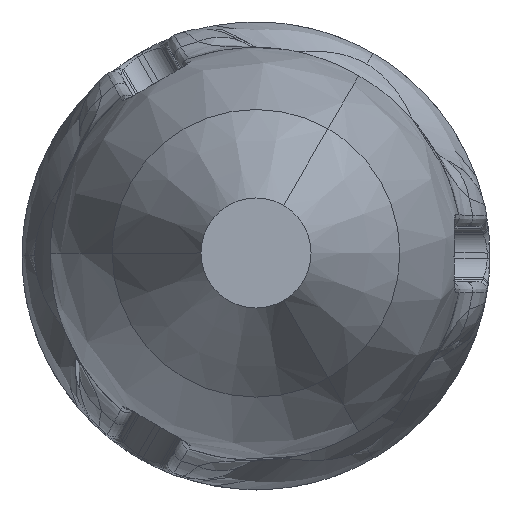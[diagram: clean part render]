
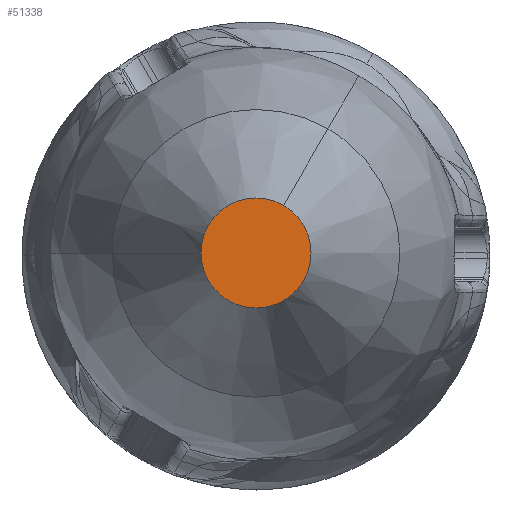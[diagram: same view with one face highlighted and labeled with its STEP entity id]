
A CAD part, top view. The second image highlights one B-rep face of the part: STEP entity #51338.
In plain terms, the highlighted planar face has unit normal (0, 0, 1).
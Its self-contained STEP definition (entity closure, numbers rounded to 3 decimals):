
#40723 = CONICAL_SURFACE('',#40724,15.,0.43);
#40724 = AXIS2_PLACEMENT_3D('',#40725,#40726,#40727);
#40725 = CARTESIAN_POINT('',(0.,0.,105.));
#40726 = DIRECTION('',(0.,0.,-1.));
#40727 = DIRECTION('',(-0.5,0.866,0.));
#42146 = CONICAL_SURFACE('',#42147,15.,0.43);
#42147 = AXIS2_PLACEMENT_3D('',#42148,#42149,#42150);
#42148 = CARTESIAN_POINT('',(0.,0.,105.));
#42149 = DIRECTION('',(0.,0.,-1.));
#42150 = DIRECTION('',(-0.5,-0.866,0.));
#47327 = CONICAL_SURFACE('',#47328,15.,0.43);
#47328 = AXIS2_PLACEMENT_3D('',#47329,#47330,#47331);
#47329 = CARTESIAN_POINT('',(0.,0.,105.));
#47330 = DIRECTION('',(-0.,0.,-1.));
#47331 = DIRECTION('',(1.,0.,0.));
#47983 = VERTEX_POINT('',#47984);
#47984 = CARTESIAN_POINT('',(-4.,0.,129.));
#48005 = VERTEX_POINT('',#48006);
#48006 = CARTESIAN_POINT('',(2.,-3.464,129.));
#48025 = EDGE_CURVE('',#47983,#48005,#48026,.T.);
#48026 = SURFACE_CURVE('',#48027,(#48032,#48039),.PCURVE_S1.);
#48027 = CIRCLE('',#48028,4.);
#48028 = AXIS2_PLACEMENT_3D('',#48029,#48030,#48031);
#48029 = CARTESIAN_POINT('',(0.,0.,129.));
#48030 = DIRECTION('',(0.,0.,1.));
#48031 = DIRECTION('',(-0.5,0.866,0.));
#48032 = PCURVE('',#40723,#48033);
#48033 = DEFINITIONAL_REPRESENTATION('',(#48034),#48038);
#48034 = LINE('',#48035,#48036);
#48035 = CARTESIAN_POINT('',(-0.,-24.));
#48036 = VECTOR('',#48037,1.);
#48037 = DIRECTION('',(-1.,-0.));
#48038 = ( GEOMETRIC_REPRESENTATION_CONTEXT(2) 
PARAMETRIC_REPRESENTATION_CONTEXT() REPRESENTATION_CONTEXT('2D SPACE',''
  ) );
#48039 = PCURVE('',#48040,#48045);
#48040 = PLANE('',#48041);
#48041 = AXIS2_PLACEMENT_3D('',#48042,#48043,#48044);
#48042 = CARTESIAN_POINT('',(0.,0.,129.));
#48043 = DIRECTION('',(0.,0.,1.));
#48044 = DIRECTION('',(0.,1.,0.));
#48045 = DEFINITIONAL_REPRESENTATION('',(#48046),#48050);
#48046 = CIRCLE('',#48047,4.);
#48047 = AXIS2_PLACEMENT_2D('',#48048,#48049);
#48048 = CARTESIAN_POINT('',(0.,0.));
#48049 = DIRECTION('',(0.866,0.5));
#48050 = ( GEOMETRIC_REPRESENTATION_CONTEXT(2) 
PARAMETRIC_REPRESENTATION_CONTEXT() REPRESENTATION_CONTEXT('2D SPACE',''
  ) );
#48536 = VERTEX_POINT('',#48537);
#48537 = CARTESIAN_POINT('',(2.,3.464,129.));
#48556 = EDGE_CURVE('',#48005,#48536,#48557,.T.);
#48557 = SURFACE_CURVE('',#48558,(#48563,#48570),.PCURVE_S1.);
#48558 = CIRCLE('',#48559,4.);
#48559 = AXIS2_PLACEMENT_3D('',#48560,#48561,#48562);
#48560 = CARTESIAN_POINT('',(0.,0.,129.));
#48561 = DIRECTION('',(0.,0.,1.));
#48562 = DIRECTION('',(-0.5,-0.866,0.));
#48563 = PCURVE('',#42146,#48564);
#48564 = DEFINITIONAL_REPRESENTATION('',(#48565),#48569);
#48565 = LINE('',#48566,#48567);
#48566 = CARTESIAN_POINT('',(-0.,-24.));
#48567 = VECTOR('',#48568,1.);
#48568 = DIRECTION('',(-1.,-0.));
#48569 = ( GEOMETRIC_REPRESENTATION_CONTEXT(2) 
PARAMETRIC_REPRESENTATION_CONTEXT() REPRESENTATION_CONTEXT('2D SPACE',''
  ) );
#48570 = PCURVE('',#48040,#48571);
#48571 = DEFINITIONAL_REPRESENTATION('',(#48572),#48576);
#48572 = CIRCLE('',#48573,4.);
#48573 = AXIS2_PLACEMENT_2D('',#48574,#48575);
#48574 = CARTESIAN_POINT('',(0.,0.));
#48575 = DIRECTION('',(-0.866,0.5));
#48576 = ( GEOMETRIC_REPRESENTATION_CONTEXT(2) 
PARAMETRIC_REPRESENTATION_CONTEXT() REPRESENTATION_CONTEXT('2D SPACE',''
  ) );
#50565 = EDGE_CURVE('',#48536,#47983,#50566,.T.);
#50566 = SURFACE_CURVE('',#50567,(#50572,#50579),.PCURVE_S1.);
#50567 = CIRCLE('',#50568,4.);
#50568 = AXIS2_PLACEMENT_3D('',#50569,#50570,#50571);
#50569 = CARTESIAN_POINT('',(0.,0.,129.));
#50570 = DIRECTION('',(-0.,0.,1.));
#50571 = DIRECTION('',(1.,0.,0.));
#50572 = PCURVE('',#47327,#50573);
#50573 = DEFINITIONAL_REPRESENTATION('',(#50574),#50578);
#50574 = LINE('',#50575,#50576);
#50575 = CARTESIAN_POINT('',(-0.,-24.));
#50576 = VECTOR('',#50577,1.);
#50577 = DIRECTION('',(-1.,-0.));
#50578 = ( GEOMETRIC_REPRESENTATION_CONTEXT(2) 
PARAMETRIC_REPRESENTATION_CONTEXT() REPRESENTATION_CONTEXT('2D SPACE',''
  ) );
#50579 = PCURVE('',#48040,#50580);
#50580 = DEFINITIONAL_REPRESENTATION('',(#50581),#50585);
#50581 = CIRCLE('',#50582,4.);
#50582 = AXIS2_PLACEMENT_2D('',#50583,#50584);
#50583 = CARTESIAN_POINT('',(0.,0.));
#50584 = DIRECTION('',(0.,-1.));
#50585 = ( GEOMETRIC_REPRESENTATION_CONTEXT(2) 
PARAMETRIC_REPRESENTATION_CONTEXT() REPRESENTATION_CONTEXT('2D SPACE',''
  ) );
#51338 = ADVANCED_FACE('',(#51339),#48040,.T.);
#51339 = FACE_BOUND('',#51340,.T.);
#51340 = EDGE_LOOP('',(#51341,#51342,#51343));
#51341 = ORIENTED_EDGE('',*,*,#48025,.T.);
#51342 = ORIENTED_EDGE('',*,*,#48556,.T.);
#51343 = ORIENTED_EDGE('',*,*,#50565,.T.);
